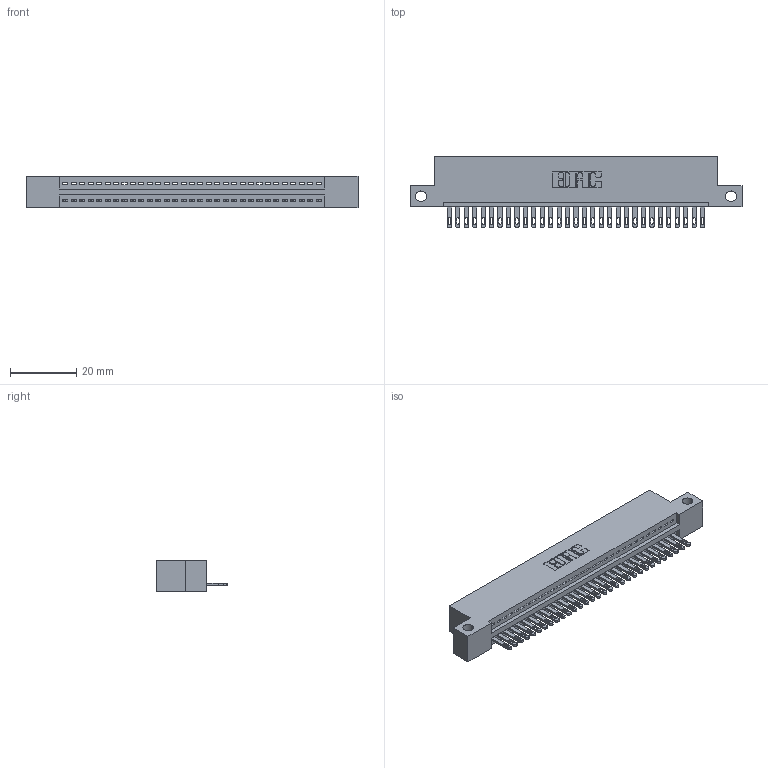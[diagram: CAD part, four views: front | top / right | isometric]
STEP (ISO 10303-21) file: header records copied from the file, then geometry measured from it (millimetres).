
FILE_DESCRIPTION (( 'STEP AP203' ), '1' );
FILE_NAME ('345-031-500-112.STEP', '2018-08-23T08:53:39', ( '' ), ( '' ), 'SwSTEP 2.0', 'SolidWorks 2016', '' );
FILE_SCHEMA (( 'CONFIG_CONTROL_DESIGN' ));
Length unit declared in the file: inch
Products named in the file (3): 345-031-500-112; 345 Part_Flush Mounting Lugs - Side Mount; 345-292-001_345-293-100
Assembly tree (32 placements, depth 2):
  345-031-500-112
    345 Part_Flush Mounting Lugs - Side Mount
    345-292-001_345-293-100  x31
Bounding box: 99.95 x 21.51 x 9.4 mm (x, y, z)
Volume: 9335 mm3; surface area: 12183.6 mm2
Topology: 32 solids, 32 shells, 1800 faces, 5549 edges, 3698 vertices
Faces by surface type: plane 1134, cylinder 666
Entity records: 24745 total; most frequent: CARTESIAN_POINT 4293, ORIENTED_EDGE 4258, DIRECTION 3767, EDGE_CURVE 2129, LINE 1869, VECTOR 1869, VERTEX_POINT 1418, AXIS2_PLACEMENT_3D 949
